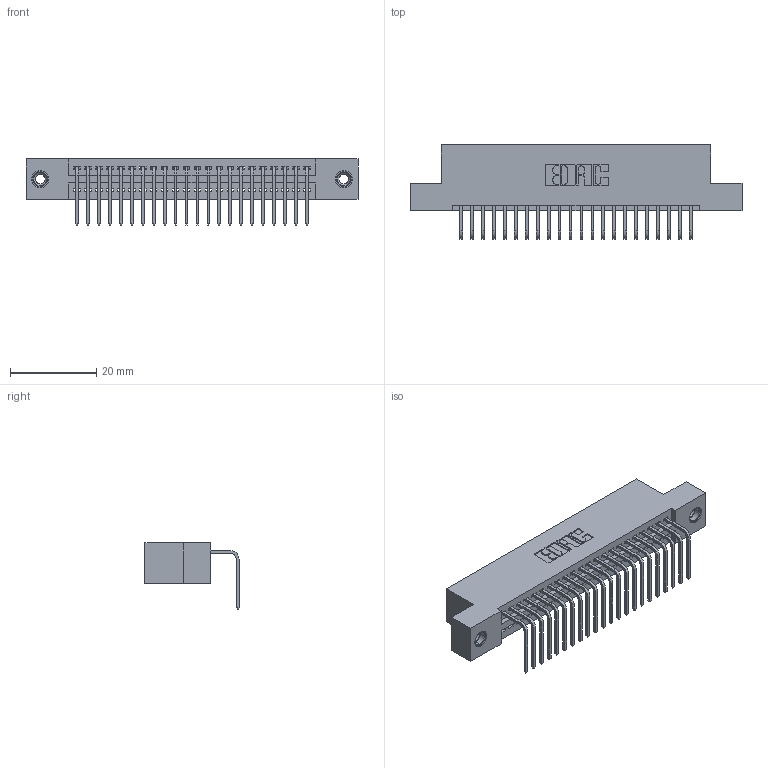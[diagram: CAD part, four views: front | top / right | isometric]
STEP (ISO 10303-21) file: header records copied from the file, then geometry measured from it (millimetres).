
FILE_DESCRIPTION (( 'STEP AP203' ), '1' );
FILE_NAME ('345-022-558-108.STEP', '2018-08-21T00:47:18', ( '' ), ( '' ), 'SwSTEP 2.0', 'SolidWorks 2016', '' );
FILE_SCHEMA (( 'CONFIG_CONTROL_DESIGN' ));
Length unit declared in the file: inch
Products named in the file (4): 345-250-001_345-250-003-102; 345-022-558-108; 345 Part_Flush Mounting Lugs - 0.156 Dia-TI; 345-292-001_558 Tail - 2
Assembly tree (25 placements, depth 2):
  345-022-558-108
    345 Part_Flush Mounting Lugs - 0.156 Dia-TI
    345-292-001_558 Tail - 2  x22
    345-250-001_345-250-003-102  x2
Bounding box: 77.09 x 21.83 x 15.37 mm (x, y, z)
Volume: 7224.9 mm3; surface area: 9779.3 mm2
Topology: 25 solids, 25 shells, 1506 faces, 4481 edges, 2950 vertices
Faces by surface type: plane 1036, cylinder 454, cone 12, torus 4
Entity records: 20520 total; most frequent: CARTESIAN_POINT 3537, ORIENTED_EDGE 3486, DIRECTION 3145, EDGE_CURVE 1743, VECTOR 1503, LINE 1503, VERTEX_POINT 1156, AXIS2_PLACEMENT_3D 821
